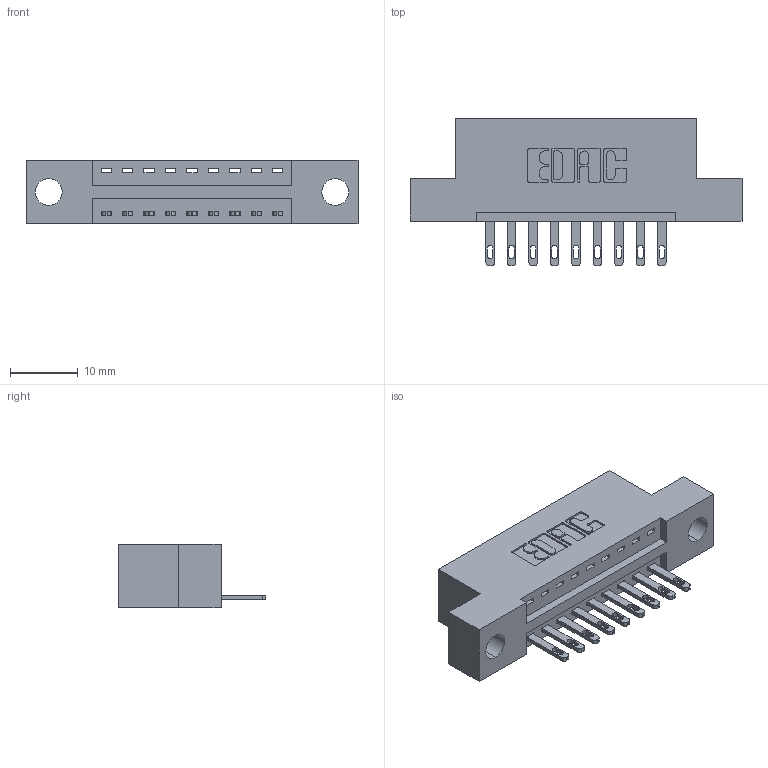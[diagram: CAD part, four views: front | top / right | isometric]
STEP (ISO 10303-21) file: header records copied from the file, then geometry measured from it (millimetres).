
FILE_DESCRIPTION (( 'STEP AP203' ), '1' );
FILE_NAME ('346-009-500-104.STEP', '2018-08-17T05:14:30', ( '' ), ( '' ), 'SwSTEP 2.0', 'SolidWorks 2016', '' );
FILE_SCHEMA (( 'CONFIG_CONTROL_DESIGN' ));
Length unit declared in the file: inch
Products named in the file (3): 346-009-500-104; 346 Part_Flush Mounting Lugs - 0.156 Dia-TH; 345-292-001_345-293-100
Assembly tree (10 placements, depth 2):
  346-009-500-104
    346 Part_Flush Mounting Lugs - 0.156 Dia-TH
    345-292-001_345-293-100  x9
Bounding box: 49.15 x 21.84 x 9.4 mm (x, y, z)
Volume: 4395 mm3; surface area: 4963 mm2
Topology: 10 solids, 10 shells, 608 faces, 1841 edges, 1226 vertices
Faces by surface type: plane 382, cylinder 226
Entity records: 9961 total; most frequent: CARTESIAN_POINT 1723, ORIENTED_EDGE 1666, DIRECTION 1563, EDGE_CURVE 833, LINE 661, VECTOR 661, VERTEX_POINT 554, AXIS2_PLACEMENT_3D 451
